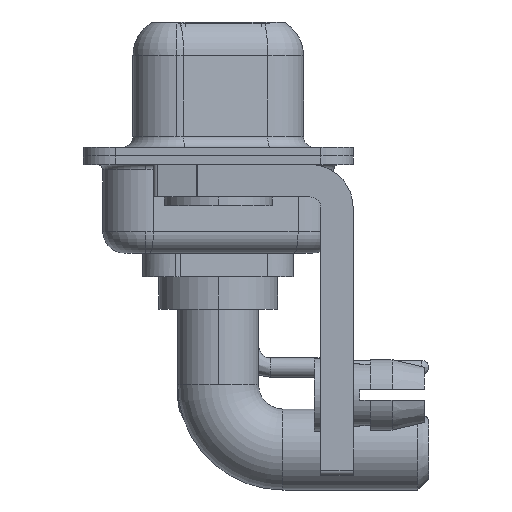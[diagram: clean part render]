
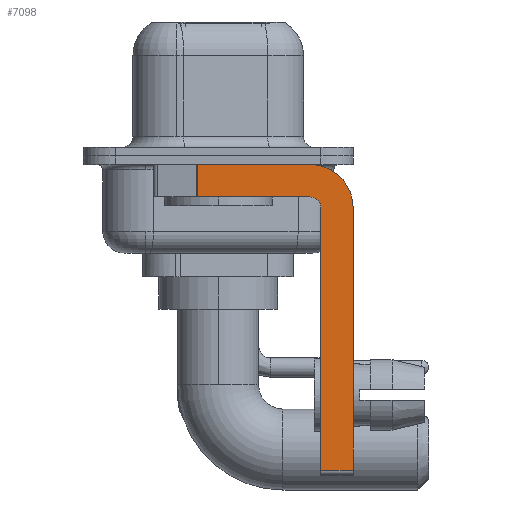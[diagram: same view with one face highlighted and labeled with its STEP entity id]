
A CAD part, left-side view. The second image highlights one B-rep face of the part: STEP entity #7098.
In plain terms, the highlighted planar face has unit normal (-1, 0, 0).
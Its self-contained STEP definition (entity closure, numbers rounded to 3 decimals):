
#91 = VERTEX_POINT ( 'NONE', #20444 ) ;
#455 = DIRECTION ( 'NONE',  ( 0., 0., -1. ) ) ;
#764 = AXIS2_PLACEMENT_3D ( 'NONE', #14655, #1714, #1820 ) ;
#1384 = CARTESIAN_POINT ( 'NONE',  ( -2.9, 3., -0.4 ) ) ;
#1714 = DIRECTION ( 'NONE',  ( 1., 0., 0. ) ) ;
#1820 = DIRECTION ( 'NONE',  ( 0., 0., -1. ) ) ;
#1989 = CARTESIAN_POINT ( 'NONE',  ( -2.9, -4.25, -0.4 ) ) ;
#2017 = EDGE_LOOP ( 'NONE', ( #9083, #14841, #12524, #13175, #9098, #19024, #21014, #8450 ) ) ;
#2294 = DIRECTION ( 'NONE',  ( 0., 0., 1. ) ) ;
#2707 = FACE_OUTER_BOUND ( 'NONE', #2017, .T. ) ;
#3150 = EDGE_CURVE ( 'NONE', #10746, #9673, #9666, .T. ) ;
#3159 = EDGE_CURVE ( 'NONE', #9463, #91, #6605, .T. ) ;
#4068 = DIRECTION ( 'NONE',  ( 0., -1., 0. ) ) ;
#4212 = CARTESIAN_POINT ( 'NONE',  ( -2.9, -4.25, -2.4 ) ) ;
#4722 = CARTESIAN_POINT ( 'NONE',  ( -2.9, 0.978, -0.4 ) ) ;
#5124 = EDGE_CURVE ( 'NONE', #15208, #10779, #9075, .T. ) ;
#5676 = DIRECTION ( 'NONE',  ( 0., 0., -1. ) ) ;
#5737 = DIRECTION ( 'NONE',  ( -1., 0., 0. ) ) ;
#6533 = AXIS2_PLACEMENT_3D ( 'NONE', #4212, #5737, #13985 ) ;
#6605 = LINE ( 'NONE', #8041, #17687 ) ;
#7098 = ADVANCED_FACE ( 'NONE', ( #2707 ), #9349, .F. ) ;
#8041 = CARTESIAN_POINT ( 'NONE',  ( -2.9, -4.25, -1.9 ) ) ;
#8450 = ORIENTED_EDGE ( 'NONE', *, *, #16283, .F. ) ;
#8662 = VECTOR ( 'NONE', #4068, 1000. ) ;
#9075 = LINE ( 'NONE', #11028, #8662 ) ;
#9083 = ORIENTED_EDGE ( 'NONE', *, *, #3150, .F. ) ;
#9098 = ORIENTED_EDGE ( 'NONE', *, *, #14903, .F. ) ;
#9349 = PLANE ( 'NONE',  #764 ) ;
#9463 = VERTEX_POINT ( 'NONE', #14610 ) ;
#9666 = LINE ( 'NONE', #1384, #13367 ) ;
#9673 = VERTEX_POINT ( 'NONE', #1989 ) ;
#9799 = CARTESIAN_POINT ( 'NONE',  ( -2.9, -4.75, -14.55 ) ) ;
#10294 = VERTEX_POINT ( 'NONE', #11093 ) ;
#10563 = LINE ( 'NONE', #17146, #16850 ) ;
#10746 = VERTEX_POINT ( 'NONE', #4722 ) ;
#10779 = VERTEX_POINT ( 'NONE', #16540 ) ;
#11028 = CARTESIAN_POINT ( 'NONE',  ( -2.9, -4.25, -14.55 ) ) ;
#11044 = VECTOR ( 'NONE', #455, 1000. ) ;
#11093 = CARTESIAN_POINT ( 'NONE',  ( -2.9, -4.75, -2.4 ) ) ;
#11393 = CIRCLE ( 'NONE', #12430, 2. ) ;
#12110 = EDGE_CURVE ( 'NONE', #10746, #91, #20588, .T. ) ;
#12430 = AXIS2_PLACEMENT_3D ( 'NONE', #20516, #20616, #5676 ) ;
#12524 = ORIENTED_EDGE ( 'NONE', *, *, #3159, .F. ) ;
#13112 = DIRECTION ( 'NONE',  ( 0., -1., 0. ) ) ;
#13175 = ORIENTED_EDGE ( 'NONE', *, *, #21181, .F. ) ;
#13367 = VECTOR ( 'NONE', #13112, 1000. ) ;
#13985 = DIRECTION ( 'NONE',  ( 0., 0., 1. ) ) ;
#14610 = CARTESIAN_POINT ( 'NONE',  ( -2.9, -4.25, -1.9 ) ) ;
#14650 = DIRECTION ( 'NONE',  ( 0., 1., 0. ) ) ;
#14655 = CARTESIAN_POINT ( 'NONE',  ( -2.9, -4.25, -2.4 ) ) ;
#14841 = ORIENTED_EDGE ( 'NONE', *, *, #12110, .T. ) ;
#14903 = EDGE_CURVE ( 'NONE', #15208, #10294, #10563, .T. ) ;
#15208 = VERTEX_POINT ( 'NONE', #9799 ) ;
#16154 = EDGE_CURVE ( 'NONE', #16406, #10779, #21387, .T. ) ;
#16244 = CIRCLE ( 'NONE', #6533, 0.5 ) ;
#16283 = EDGE_CURVE ( 'NONE', #9673, #16406, #11393, .T. ) ;
#16406 = VERTEX_POINT ( 'NONE', #19118 ) ;
#16540 = CARTESIAN_POINT ( 'NONE',  ( -2.9, -6.25, -14.55 ) ) ;
#16850 = VECTOR ( 'NONE', #2294, 1000. ) ;
#17146 = CARTESIAN_POINT ( 'NONE',  ( -2.9, -4.75, -14.8 ) ) ;
#17687 = VECTOR ( 'NONE', #14650, 1000. ) ;
#18860 = DIRECTION ( 'NONE',  ( 0., 0., -1. ) ) ;
#19024 = ORIENTED_EDGE ( 'NONE', *, *, #5124, .T. ) ;
#19118 = CARTESIAN_POINT ( 'NONE',  ( -2.9, -6.25, -2.4 ) ) ;
#19591 = VECTOR ( 'NONE', #18860, 1000. ) ;
#20199 = CARTESIAN_POINT ( 'NONE',  ( -2.9, -6.25, -2.4 ) ) ;
#20444 = CARTESIAN_POINT ( 'NONE',  ( -2.9, 0.978, -1.9 ) ) ;
#20516 = CARTESIAN_POINT ( 'NONE',  ( -2.9, -4.25, -2.4 ) ) ;
#20588 = LINE ( 'NONE', #20813, #19591 ) ;
#20616 = DIRECTION ( 'NONE',  ( 1., 0., 0. ) ) ;
#20813 = CARTESIAN_POINT ( 'NONE',  ( -2.9, 0.978, -1.9 ) ) ;
#21014 = ORIENTED_EDGE ( 'NONE', *, *, #16154, .F. ) ;
#21181 = EDGE_CURVE ( 'NONE', #10294, #9463, #16244, .T. ) ;
#21387 = LINE ( 'NONE', #20199, #11044 ) ;
